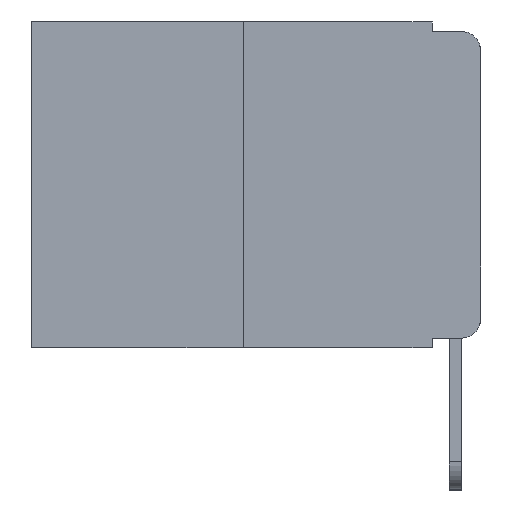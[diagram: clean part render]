
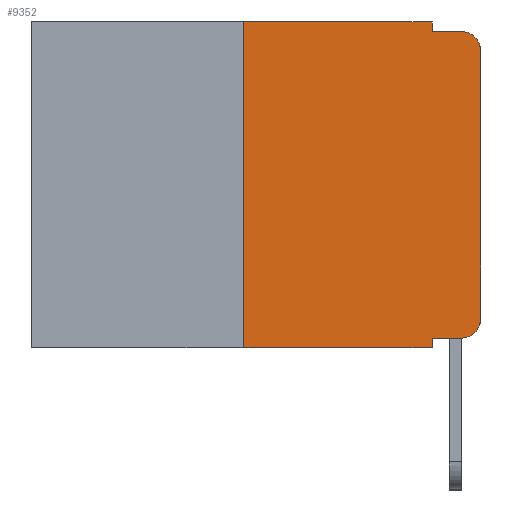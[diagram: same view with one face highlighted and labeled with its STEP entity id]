
A CAD part, left-side view. The second image highlights one B-rep face of the part: STEP entity #9352.
In plain terms, the highlighted planar face has unit normal (-1, 0, 0).
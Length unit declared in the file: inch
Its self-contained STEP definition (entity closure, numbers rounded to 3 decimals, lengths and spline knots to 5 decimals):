
#239 = VERTEX_POINT ( 'NONE', #748 ) ;
#346 = LINE ( 'NONE', #4530, #12574 ) ;
#368 = VERTEX_POINT ( 'NONE', #9448 ) ;
#372 = ORIENTED_EDGE ( 'NONE', *, *, #4050, .T. ) ;
#732 = VECTOR ( 'NONE', #10993, 39.37008 ) ;
#748 = CARTESIAN_POINT ( 'NONE',  ( 0., 0.02, -0.01 ) ) ;
#764 = DIRECTION ( 'NONE',  ( -1., 0., 0. ) ) ;
#911 = ORIENTED_EDGE ( 'NONE', *, *, #4001, .F. ) ;
#1153 = ORIENTED_EDGE ( 'NONE', *, *, #3922, .T. ) ;
#1188 = ORIENTED_EDGE ( 'NONE', *, *, #3239, .F. ) ;
#1276 = ORIENTED_EDGE ( 'NONE', *, *, #3962, .F. ) ;
#1732 = ORIENTED_EDGE ( 'NONE', *, *, #4007, .F. ) ;
#1772 = DIRECTION ( 'NONE',  ( 0., 0., -1. ) ) ;
#1881 = EDGE_LOOP ( 'NONE', ( #1153, #5669, #1276, #911, #1188, #1732, #5368, #6212, #11177, #372 ) ) ;
#2311 = CARTESIAN_POINT ( 'NONE',  ( 0., 0.051, 0. ) ) ;
#2329 = CARTESIAN_POINT ( 'NONE',  ( 0., 0.051, -0.333 ) ) ;
#2419 = DIRECTION ( 'NONE',  ( 0., 0., 1. ) ) ;
#2687 = CIRCLE ( 'NONE', #9800, 0.02 ) ;
#2701 = DIRECTION ( 'NONE',  ( 0., -1., 0. ) ) ;
#2830 = CARTESIAN_POINT ( 'NONE',  ( 0., 0.473, 0. ) ) ;
#3057 = VECTOR ( 'NONE', #12348, 39.37008 ) ;
#3149 = VERTEX_POINT ( 'NONE', #4504 ) ;
#3239 = EDGE_CURVE ( 'NONE', #10924, #9563, #7268, .T. ) ;
#3279 = DIRECTION ( 'NONE',  ( 0., -1., 0. ) ) ;
#3453 = DIRECTION ( 'NONE',  ( 0., -1., 0. ) ) ;
#3584 = VECTOR ( 'NONE', #5523, 39.37008 ) ;
#3610 = CARTESIAN_POINT ( 'NONE',  ( 0., 0.473, 0. ) ) ;
#3622 = EDGE_CURVE ( 'NONE', #8305, #10241, #5825, .T. ) ;
#3922 = EDGE_CURVE ( 'NONE', #8462, #3149, #5815, .T. ) ;
#3942 = EDGE_CURVE ( 'NONE', #3149, #239, #2687, .T. ) ;
#3962 = EDGE_CURVE ( 'NONE', #5340, #239, #9701, .T. ) ;
#4001 = EDGE_CURVE ( 'NONE', #9563, #5340, #4261, .T. ) ;
#4007 = EDGE_CURVE ( 'NONE', #8305, #10924, #6548, .T. ) ;
#4027 = EDGE_CURVE ( 'NONE', #6651, #10241, #8934, .T. ) ;
#4045 = EDGE_CURVE ( 'NONE', #6651, #368, #346, .T. ) ;
#4050 = EDGE_CURVE ( 'NONE', #368, #8462, #8384, .T. ) ;
#4261 = LINE ( 'NONE', #5687, #9208 ) ;
#4444 = VECTOR ( 'NONE', #2701, 39.37008 ) ;
#4504 = CARTESIAN_POINT ( 'NONE',  ( 0., 0., -0.03 ) ) ;
#4530 = CARTESIAN_POINT ( 'NONE',  ( 0., 0.051, -0.333 ) ) ;
#4951 = CARTESIAN_POINT ( 'NONE',  ( 0., 0.473, -0.343 ) ) ;
#5340 = VERTEX_POINT ( 'NONE', #7000 ) ;
#5368 = ORIENTED_EDGE ( 'NONE', *, *, #3622, .T. ) ;
#5400 = CARTESIAN_POINT ( 'NONE',  ( 0., 0.25, -0.343 ) ) ;
#5523 = DIRECTION ( 'NONE',  ( 0., 0., -1. ) ) ;
#5669 = ORIENTED_EDGE ( 'NONE', *, *, #3942, .T. ) ;
#5687 = CARTESIAN_POINT ( 'NONE',  ( 0., 0.051, 0. ) ) ;
#5815 = LINE ( 'NONE', #8377, #12201 ) ;
#5825 = LINE ( 'NONE', #4951, #3057 ) ;
#6035 = DIRECTION ( 'NONE',  ( 0., 0., -1. ) ) ;
#6212 = ORIENTED_EDGE ( 'NONE', *, *, #4027, .F. ) ;
#6548 = LINE ( 'NONE', #6626, #732 ) ;
#6603 = DIRECTION ( 'NONE',  ( 1., 0., 0. ) ) ;
#6626 = CARTESIAN_POINT ( 'NONE',  ( 0., 0.25, 0. ) ) ;
#6651 = VERTEX_POINT ( 'NONE', #2329 ) ;
#7000 = CARTESIAN_POINT ( 'NONE',  ( 0., 0.051, -0.01 ) ) ;
#7120 = AXIS2_PLACEMENT_3D ( 'NONE', #3610, #6603, #6035 ) ;
#7186 = CARTESIAN_POINT ( 'NONE',  ( 0., 0.051, -0.01 ) ) ;
#7268 = LINE ( 'NONE', #2830, #4444 ) ;
#7443 = CARTESIAN_POINT ( 'NONE',  ( 0., 0.02, -0.03 ) ) ;
#7551 = DIRECTION ( 'NONE',  ( 0., 0., -1. ) ) ;
#7670 = CARTESIAN_POINT ( 'NONE',  ( 0., 0.25, 0. ) ) ;
#8305 = VERTEX_POINT ( 'NONE', #5400 ) ;
#8377 = CARTESIAN_POINT ( 'NONE',  ( 0., 0., 0. ) ) ;
#8384 = CIRCLE ( 'NONE', #9136, 0.02 ) ;
#8422 = FACE_OUTER_BOUND ( 'NONE', #1881, .T. ) ;
#8462 = VERTEX_POINT ( 'NONE', #11781 ) ;
#8934 = LINE ( 'NONE', #2311, #3584 ) ;
#9136 = AXIS2_PLACEMENT_3D ( 'NONE', #10896, #10050, #9263 ) ;
#9208 = VECTOR ( 'NONE', #7551, 39.37008 ) ;
#9263 = DIRECTION ( 'NONE',  ( 0., 0., -1. ) ) ;
#9352 = ADVANCED_FACE ( 'NONE', ( #8422 ), #11778, .F. ) ;
#9448 = CARTESIAN_POINT ( 'NONE',  ( 0., 0.02, -0.333 ) ) ;
#9563 = VERTEX_POINT ( 'NONE', #11984 ) ;
#9701 = LINE ( 'NONE', #7186, #11690 ) ;
#9800 = AXIS2_PLACEMENT_3D ( 'NONE', #7443, #764, #1772 ) ;
#10050 = DIRECTION ( 'NONE',  ( -1., 0., 0. ) ) ;
#10241 = VERTEX_POINT ( 'NONE', #11869 ) ;
#10896 = CARTESIAN_POINT ( 'NONE',  ( 0., 0.02, -0.313 ) ) ;
#10924 = VERTEX_POINT ( 'NONE', #7670 ) ;
#10993 = DIRECTION ( 'NONE',  ( 0., 0., 1. ) ) ;
#11177 = ORIENTED_EDGE ( 'NONE', *, *, #4045, .T. ) ;
#11690 = VECTOR ( 'NONE', #3279, 39.37008 ) ;
#11778 = PLANE ( 'NONE',  #7120 ) ;
#11781 = CARTESIAN_POINT ( 'NONE',  ( 0., 0., -0.313 ) ) ;
#11869 = CARTESIAN_POINT ( 'NONE',  ( 0., 0.051, -0.343 ) ) ;
#11984 = CARTESIAN_POINT ( 'NONE',  ( 0., 0.051, 0. ) ) ;
#12201 = VECTOR ( 'NONE', #2419, 39.37008 ) ;
#12348 = DIRECTION ( 'NONE',  ( 0., -1., 0. ) ) ;
#12574 = VECTOR ( 'NONE', #3453, 39.37008 ) ;
